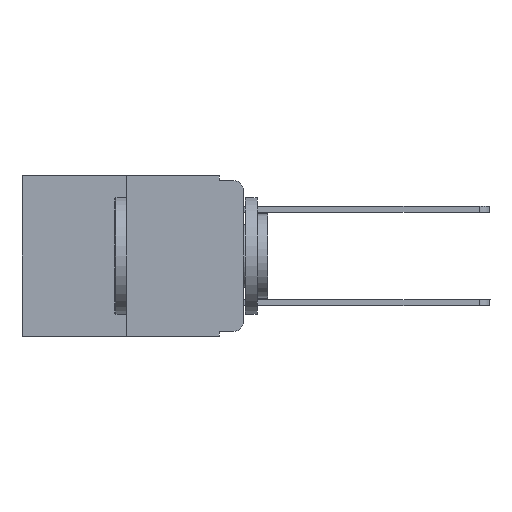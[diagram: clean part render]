
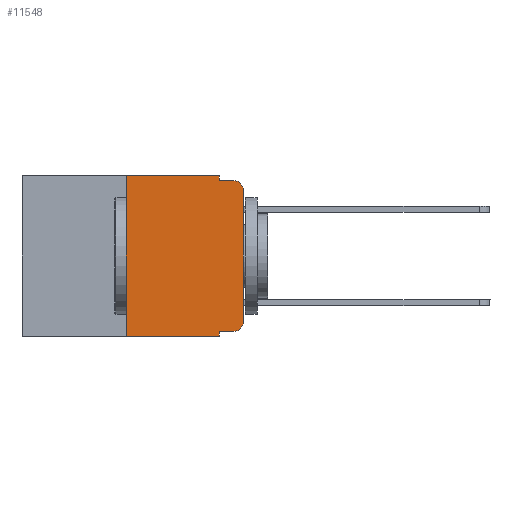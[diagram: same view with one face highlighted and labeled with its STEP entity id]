
A CAD part, left-side view. The second image highlights one B-rep face of the part: STEP entity #11548.
In plain terms, the highlighted planar face has unit normal (-1, 0, 0).
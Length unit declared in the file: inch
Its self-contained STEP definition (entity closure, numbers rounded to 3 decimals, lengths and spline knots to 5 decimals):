
#50 = DIRECTION ( 'NONE',  ( 0., -1., 0. ) ) ;
#134 = FACE_OUTER_BOUND ( 'NONE', #5957, .T. ) ;
#176 = EDGE_CURVE ( 'NONE', #3535, #3271, #711, .T. ) ;
#228 = CARTESIAN_POINT ( 'NONE',  ( 0., 0.473, 0. ) ) ;
#351 = AXIS2_PLACEMENT_3D ( 'NONE', #6678, #586, #1604 ) ;
#427 = CARTESIAN_POINT ( 'NONE',  ( 0., 0.051, 0. ) ) ;
#443 = VERTEX_POINT ( 'NONE', #4571 ) ;
#561 = ORIENTED_EDGE ( 'NONE', *, *, #11879, .T. ) ;
#562 = VERTEX_POINT ( 'NONE', #9309 ) ;
#586 = DIRECTION ( 'NONE',  ( -1., 0., 0. ) ) ;
#711 = CIRCLE ( 'NONE', #10333, 0.02 ) ;
#822 = CARTESIAN_POINT ( 'NONE',  ( 0., 0., 0. ) ) ;
#991 = CARTESIAN_POINT ( 'NONE',  ( 0., 0.051, -0.333 ) ) ;
#1262 = VECTOR ( 'NONE', #50, 39.37008 ) ;
#1604 = DIRECTION ( 'NONE',  ( 0., 0., -1. ) ) ;
#1701 = DIRECTION ( 'NONE',  ( 0., -1., 0. ) ) ;
#1880 = ORIENTED_EDGE ( 'NONE', *, *, #12703, .F. ) ;
#1884 = VERTEX_POINT ( 'NONE', #9773 ) ;
#1909 = CARTESIAN_POINT ( 'NONE',  ( 0., 0., -0.03 ) ) ;
#2007 = EDGE_CURVE ( 'NONE', #7686, #1884, #9872, .T. ) ;
#2065 = LINE ( 'NONE', #8150, #3677 ) ;
#2191 = ORIENTED_EDGE ( 'NONE', *, *, #5032, .T. ) ;
#2215 = CARTESIAN_POINT ( 'NONE',  ( 0., 0.051, -0.01 ) ) ;
#2238 = DIRECTION ( 'NONE',  ( 1., 0., 0. ) ) ;
#2330 = DIRECTION ( 'NONE',  ( 0., 0., 1. ) ) ;
#2503 = DIRECTION ( 'NONE',  ( 0., 0., -1. ) ) ;
#2964 = CARTESIAN_POINT ( 'NONE',  ( 0., 0.051, 0. ) ) ;
#2988 = EDGE_CURVE ( 'NONE', #6135, #12549, #2065, .T. ) ;
#3257 = DIRECTION ( 'NONE',  ( 0., -1., 0. ) ) ;
#3271 = VERTEX_POINT ( 'NONE', #5439 ) ;
#3375 = ORIENTED_EDGE ( 'NONE', *, *, #11310, .T. ) ;
#3515 = LINE ( 'NONE', #991, #1262 ) ;
#3535 = VERTEX_POINT ( 'NONE', #1909 ) ;
#3677 = VECTOR ( 'NONE', #1701, 39.37008 ) ;
#3833 = ORIENTED_EDGE ( 'NONE', *, *, #6924, .F. ) ;
#3979 = CARTESIAN_POINT ( 'NONE',  ( 0., 0.051, 0. ) ) ;
#4360 = CARTESIAN_POINT ( 'NONE',  ( 0., 0.25, 0. ) ) ;
#4425 = LINE ( 'NONE', #822, #9503 ) ;
#4571 = CARTESIAN_POINT ( 'NONE',  ( 0., 0.051, -0.333 ) ) ;
#4788 = EDGE_CURVE ( 'NONE', #443, #12549, #8088, .T. ) ;
#5030 = CARTESIAN_POINT ( 'NONE',  ( 0., 0.051, -0.343 ) ) ;
#5032 = EDGE_CURVE ( 'NONE', #8484, #562, #5847, .T. ) ;
#5181 = AXIS2_PLACEMENT_3D ( 'NONE', #7359, #2238, #11366 ) ;
#5251 = DIRECTION ( 'NONE',  ( 0., -1., 0. ) ) ;
#5439 = CARTESIAN_POINT ( 'NONE',  ( 0., 0.02, -0.01 ) ) ;
#5615 = DIRECTION ( 'NONE',  ( 0., 0., -1. ) ) ;
#5738 = ORIENTED_EDGE ( 'NONE', *, *, #4788, .F. ) ;
#5847 = CIRCLE ( 'NONE', #351, 0.02 ) ;
#5957 = EDGE_LOOP ( 'NONE', ( #561, #7772, #3833, #8927, #10693, #1880, #9522, #5738, #3375, #2191 ) ) ;
#5983 = DIRECTION ( 'NONE',  ( 0., 0., 1. ) ) ;
#6135 = VERTEX_POINT ( 'NONE', #11462 ) ;
#6678 = CARTESIAN_POINT ( 'NONE',  ( 0., 0.02, -0.313 ) ) ;
#6742 = CARTESIAN_POINT ( 'NONE',  ( 0., 0.02, -0.333 ) ) ;
#6924 = EDGE_CURVE ( 'NONE', #1884, #3271, #13074, .T. ) ;
#7192 = VECTOR ( 'NONE', #5615, 39.37008 ) ;
#7236 = VECTOR ( 'NONE', #2330, 39.37008 ) ;
#7311 = PLANE ( 'NONE',  #5181 ) ;
#7359 = CARTESIAN_POINT ( 'NONE',  ( 0., 0.473, 0. ) ) ;
#7562 = VECTOR ( 'NONE', #5251, 39.37008 ) ;
#7686 = VERTEX_POINT ( 'NONE', #2964 ) ;
#7772 = ORIENTED_EDGE ( 'NONE', *, *, #176, .T. ) ;
#7860 = LINE ( 'NONE', #4360, #7236 ) ;
#8046 = CARTESIAN_POINT ( 'NONE',  ( 0., 0.02, -0.03 ) ) ;
#8088 = LINE ( 'NONE', #3979, #10457 ) ;
#8150 = CARTESIAN_POINT ( 'NONE',  ( 0., 0.473, -0.343 ) ) ;
#8484 = VERTEX_POINT ( 'NONE', #6742 ) ;
#8927 = ORIENTED_EDGE ( 'NONE', *, *, #2007, .F. ) ;
#9309 = CARTESIAN_POINT ( 'NONE',  ( 0., 0., -0.313 ) ) ;
#9503 = VECTOR ( 'NONE', #5983, 39.37008 ) ;
#9522 = ORIENTED_EDGE ( 'NONE', *, *, #2988, .T. ) ;
#9773 = CARTESIAN_POINT ( 'NONE',  ( 0., 0.051, -0.01 ) ) ;
#9872 = LINE ( 'NONE', #427, #7192 ) ;
#10333 = AXIS2_PLACEMENT_3D ( 'NONE', #8046, #11701, #2503 ) ;
#10457 = VECTOR ( 'NONE', #11056, 39.37008 ) ;
#10580 = VECTOR ( 'NONE', #3257, 39.37008 ) ;
#10588 = CARTESIAN_POINT ( 'NONE',  ( 0., 0.25, 0. ) ) ;
#10693 = ORIENTED_EDGE ( 'NONE', *, *, #12674, .F. ) ;
#11056 = DIRECTION ( 'NONE',  ( 0., 0., -1. ) ) ;
#11310 = EDGE_CURVE ( 'NONE', #443, #8484, #3515, .T. ) ;
#11366 = DIRECTION ( 'NONE',  ( 0., 0., -1. ) ) ;
#11462 = CARTESIAN_POINT ( 'NONE',  ( 0., 0.25, -0.343 ) ) ;
#11548 = ADVANCED_FACE ( 'NONE', ( #134 ), #7311, .F. ) ;
#11701 = DIRECTION ( 'NONE',  ( -1., 0., 0. ) ) ;
#11879 = EDGE_CURVE ( 'NONE', #562, #3535, #4425, .T. ) ;
#12173 = VERTEX_POINT ( 'NONE', #10588 ) ;
#12549 = VERTEX_POINT ( 'NONE', #5030 ) ;
#12674 = EDGE_CURVE ( 'NONE', #12173, #7686, #12899, .T. ) ;
#12703 = EDGE_CURVE ( 'NONE', #6135, #12173, #7860, .T. ) ;
#12899 = LINE ( 'NONE', #228, #7562 ) ;
#13074 = LINE ( 'NONE', #2215, #10580 ) ;
